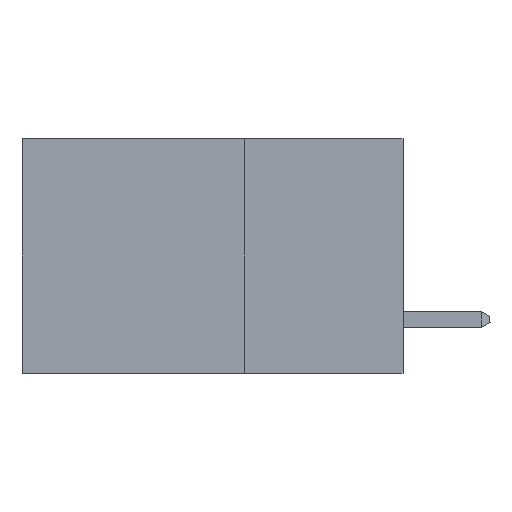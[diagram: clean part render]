
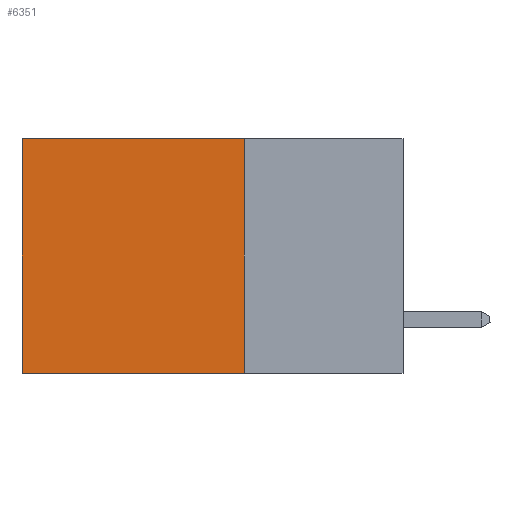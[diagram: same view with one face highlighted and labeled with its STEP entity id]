
A CAD part, left-side view. The second image highlights one B-rep face of the part: STEP entity #6351.
In plain terms, the highlighted planar face has unit normal (-1, 0, 0).
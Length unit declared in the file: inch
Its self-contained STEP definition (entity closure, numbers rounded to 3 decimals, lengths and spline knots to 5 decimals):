
#438 = VERTEX_POINT ( 'NONE', #9840 ) ;
#1523 = CARTESIAN_POINT ( 'NONE',  ( 0.2875, 0.6, -0.37 ) ) ;
#1599 = CARTESIAN_POINT ( 'NONE',  ( 0.2875, 0.6, 0. ) ) ;
#3211 = VERTEX_POINT ( 'NONE', #1599 ) ;
#3398 = EDGE_CURVE ( 'NONE', #438, #3211, #9622, .T. ) ;
#3793 = CARTESIAN_POINT ( 'NONE',  ( 0.2875, 0.6, 0. ) ) ;
#3911 = CARTESIAN_POINT ( 'NONE',  ( 0.2875, 0.25, 0. ) ) ;
#3981 = CARTESIAN_POINT ( 'NONE',  ( 0.2875, 0.25, -0.37 ) ) ;
#4071 = ORIENTED_EDGE ( 'NONE', *, *, #7616, .F. ) ;
#4196 = EDGE_LOOP ( 'NONE', ( #15683, #4071, #13310, #11128 ) ) ;
#4855 = CARTESIAN_POINT ( 'NONE',  ( 0.2875, 0.25, -0.37 ) ) ;
#5746 = DIRECTION ( 'NONE',  ( 0., 1., 0. ) ) ;
#6351 = ADVANCED_FACE ( 'NONE', ( #11006 ), #18403, .F. ) ;
#6427 = VECTOR ( 'NONE', #19825, 39.37008 ) ;
#6826 = VECTOR ( 'NONE', #5746, 39.37008 ) ;
#6980 = DIRECTION ( 'NONE',  ( 0., 0., -1. ) ) ;
#7494 = DIRECTION ( 'NONE',  ( 0., 1., 0. ) ) ;
#7616 = EDGE_CURVE ( 'NONE', #10594, #17243, #14295, .T. ) ;
#9622 = LINE ( 'NONE', #15516, #6826 ) ;
#9840 = CARTESIAN_POINT ( 'NONE',  ( 0.2875, 0.25, 0. ) ) ;
#10110 = CARTESIAN_POINT ( 'NONE',  ( 0.2875, 0.25, 0. ) ) ;
#10195 = VECTOR ( 'NONE', #7494, 39.37008 ) ;
#10594 = VERTEX_POINT ( 'NONE', #4855 ) ;
#11006 = FACE_OUTER_BOUND ( 'NONE', #4196, .T. ) ;
#11128 = ORIENTED_EDGE ( 'NONE', *, *, #3398, .T. ) ;
#13310 = ORIENTED_EDGE ( 'NONE', *, *, #20923, .F. ) ;
#14295 = LINE ( 'NONE', #3981, #10195 ) ;
#15516 = CARTESIAN_POINT ( 'NONE',  ( 0.2875, 0.25, 0. ) ) ;
#15683 = ORIENTED_EDGE ( 'NONE', *, *, #18551, .T. ) ;
#15762 = VECTOR ( 'NONE', #6980, 39.37008 ) ;
#16004 = LINE ( 'NONE', #10110, #15762 ) ;
#16114 = LINE ( 'NONE', #3793, #6427 ) ;
#16977 = DIRECTION ( 'NONE',  ( 1., 0., 0. ) ) ;
#17006 = AXIS2_PLACEMENT_3D ( 'NONE', #3911, #16977, #20091 ) ;
#17243 = VERTEX_POINT ( 'NONE', #1523 ) ;
#18403 = PLANE ( 'NONE',  #17006 ) ;
#18551 = EDGE_CURVE ( 'NONE', #3211, #17243, #16114, .T. ) ;
#19825 = DIRECTION ( 'NONE',  ( 0., 0., -1. ) ) ;
#20091 = DIRECTION ( 'NONE',  ( 0., 0., -1. ) ) ;
#20923 = EDGE_CURVE ( 'NONE', #438, #10594, #16004, .T. ) ;
